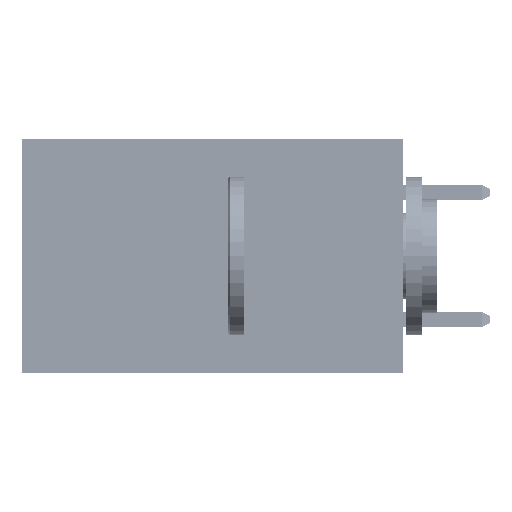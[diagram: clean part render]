
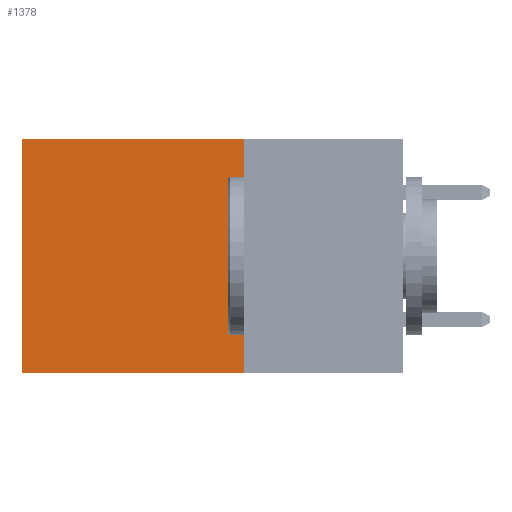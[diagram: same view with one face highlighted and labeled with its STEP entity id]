
A CAD part, left-side view. The second image highlights one B-rep face of the part: STEP entity #1378.
In plain terms, the highlighted planar face has unit normal (-1, 0, 0).
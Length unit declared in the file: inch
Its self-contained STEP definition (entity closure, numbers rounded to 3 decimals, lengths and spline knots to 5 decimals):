
#1378 = ADVANCED_FACE ( 'NONE', ( #7536 ), #31579, .F. ) ;
#2855 = DIRECTION ( 'NONE',  ( 0., 1., 0. ) ) ;
#4151 = CARTESIAN_POINT ( 'NONE',  ( 0.2875, 0.25, 0. ) ) ;
#4381 = VECTOR ( 'NONE', #41938, 39.37008 ) ;
#4865 = VERTEX_POINT ( 'NONE', #32816 ) ;
#5279 = ORIENTED_EDGE ( 'NONE', *, *, #5713, .T. ) ;
#5713 = EDGE_CURVE ( 'NONE', #29613, #4865, #27705, .T. ) ;
#7536 = FACE_OUTER_BOUND ( 'NONE', #29657, .T. ) ;
#11551 = EDGE_CURVE ( 'NONE', #17221, #4865, #40318, .T. ) ;
#13956 = DIRECTION ( 'NONE',  ( 0., 1., 0. ) ) ;
#15884 = AXIS2_PLACEMENT_3D ( 'NONE', #4151, #29236, #29855 ) ;
#16448 = VECTOR ( 'NONE', #2855, 39.37008 ) ;
#16549 = ORIENTED_EDGE ( 'NONE', *, *, #43123, .F. ) ;
#17221 = VERTEX_POINT ( 'NONE', #33284 ) ;
#18113 = LINE ( 'NONE', #27079, #34208 ) ;
#19480 = DIRECTION ( 'NONE',  ( 0., 0., -1. ) ) ;
#21828 = ORIENTED_EDGE ( 'NONE', *, *, #34455, .T. ) ;
#26919 = VERTEX_POINT ( 'NONE', #31733 ) ;
#27079 = CARTESIAN_POINT ( 'NONE',  ( 0.2875, 0.25, 0. ) ) ;
#27705 = LINE ( 'NONE', #45199, #4381 ) ;
#29236 = DIRECTION ( 'NONE',  ( 1., 0., 0. ) ) ;
#29613 = VERTEX_POINT ( 'NONE', #36087 ) ;
#29657 = EDGE_LOOP ( 'NONE', ( #5279, #31781, #16549, #21828 ) ) ;
#29855 = DIRECTION ( 'NONE',  ( 0., 0., -1. ) ) ;
#31408 = LINE ( 'NONE', #38356, #16448 ) ;
#31579 = PLANE ( 'NONE',  #15884 ) ;
#31733 = CARTESIAN_POINT ( 'NONE',  ( 0.2875, 0.25, 0. ) ) ;
#31781 = ORIENTED_EDGE ( 'NONE', *, *, #11551, .F. ) ;
#32816 = CARTESIAN_POINT ( 'NONE',  ( 0.2875, 0.6, -0.37 ) ) ;
#33284 = CARTESIAN_POINT ( 'NONE',  ( 0.2875, 0.25, -0.37 ) ) ;
#34208 = VECTOR ( 'NONE', #19480, 39.37008 ) ;
#34455 = EDGE_CURVE ( 'NONE', #26919, #29613, #31408, .T. ) ;
#34783 = VECTOR ( 'NONE', #13956, 39.37008 ) ;
#36087 = CARTESIAN_POINT ( 'NONE',  ( 0.2875, 0.6, 0. ) ) ;
#38356 = CARTESIAN_POINT ( 'NONE',  ( 0.2875, 0.25, 0. ) ) ;
#40318 = LINE ( 'NONE', #45583, #34783 ) ;
#41938 = DIRECTION ( 'NONE',  ( 0., 0., -1. ) ) ;
#43123 = EDGE_CURVE ( 'NONE', #26919, #17221, #18113, .T. ) ;
#45199 = CARTESIAN_POINT ( 'NONE',  ( 0.2875, 0.6, 0. ) ) ;
#45583 = CARTESIAN_POINT ( 'NONE',  ( 0.2875, 0.25, -0.37 ) ) ;
